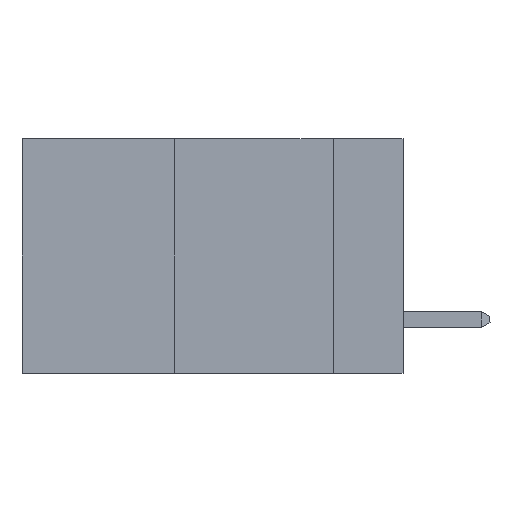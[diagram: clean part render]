
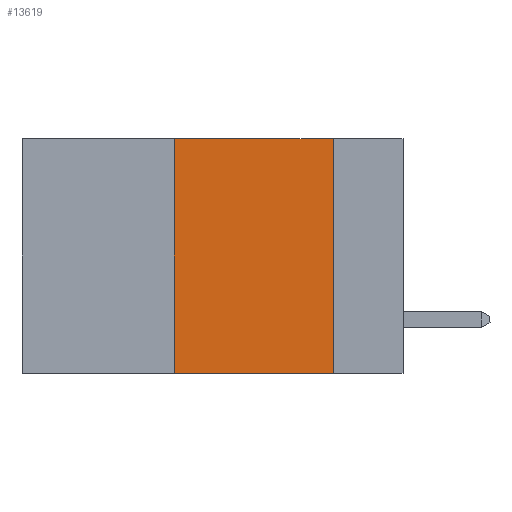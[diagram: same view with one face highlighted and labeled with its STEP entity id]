
A CAD part, left-side view. The second image highlights one B-rep face of the part: STEP entity #13619.
In plain terms, the highlighted planar face has unit normal (-1, 0, 0).
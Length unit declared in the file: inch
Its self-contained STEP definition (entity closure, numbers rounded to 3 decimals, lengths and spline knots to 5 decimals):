
#525 = DIRECTION ( 'NONE',  ( 1., 0., 0. ) ) ;
#1082 = ORIENTED_EDGE ( 'NONE', *, *, #5731, .F. ) ;
#1224 = ORIENTED_EDGE ( 'NONE', *, *, #4585, .F. ) ;
#1263 = ORIENTED_EDGE ( 'NONE', *, *, #1955, .F. ) ;
#1331 = ORIENTED_EDGE ( 'NONE', *, *, #15946, .T. ) ;
#1877 = LINE ( 'NONE', #10360, #13682 ) ;
#1931 = CARTESIAN_POINT ( 'NONE',  ( 0., 0.11, 0. ) ) ;
#1955 = EDGE_CURVE ( 'NONE', #7000, #3945, #12237, .T. ) ;
#1991 = DIRECTION ( 'NONE',  ( 0., -1., 0. ) ) ;
#2933 = AXIS2_PLACEMENT_3D ( 'NONE', #16819, #525, #10323 ) ;
#3236 = CARTESIAN_POINT ( 'NONE',  ( 0., 0.36, -0.37 ) ) ;
#3374 = FACE_OUTER_BOUND ( 'NONE', #6062, .T. ) ;
#3945 = VERTEX_POINT ( 'NONE', #11039 ) ;
#4585 = EDGE_CURVE ( 'NONE', #3945, #13025, #9209, .T. ) ;
#5635 = DIRECTION ( 'NONE',  ( 0., 0., 1. ) ) ;
#5731 = EDGE_CURVE ( 'NONE', #13025, #6872, #15547, .T. ) ;
#6062 = EDGE_LOOP ( 'NONE', ( #1082, #1224, #1263, #1331 ) ) ;
#6872 = VERTEX_POINT ( 'NONE', #16484 ) ;
#7000 = VERTEX_POINT ( 'NONE', #3236 ) ;
#8939 = PLANE ( 'NONE',  #2933 ) ;
#9209 = LINE ( 'NONE', #15872, #12745 ) ;
#9902 = CARTESIAN_POINT ( 'NONE',  ( 0., 0.36, 0. ) ) ;
#10323 = DIRECTION ( 'NONE',  ( 0., 0., -1. ) ) ;
#10360 = CARTESIAN_POINT ( 'NONE',  ( 0., 0.6, -0.37 ) ) ;
#11039 = CARTESIAN_POINT ( 'NONE',  ( 0., 0.36, 0. ) ) ;
#12016 = DIRECTION ( 'NONE',  ( 0., -1., 0. ) ) ;
#12237 = LINE ( 'NONE', #9902, #15274 ) ;
#12509 = VECTOR ( 'NONE', #12957, 39.37008 ) ;
#12745 = VECTOR ( 'NONE', #12016, 39.37008 ) ;
#12957 = DIRECTION ( 'NONE',  ( 0., 0., -1. ) ) ;
#13025 = VERTEX_POINT ( 'NONE', #16656 ) ;
#13619 = ADVANCED_FACE ( 'NONE', ( #3374 ), #8939, .F. ) ;
#13682 = VECTOR ( 'NONE', #1991, 39.37008 ) ;
#15274 = VECTOR ( 'NONE', #5635, 39.37008 ) ;
#15547 = LINE ( 'NONE', #1931, #12509 ) ;
#15872 = CARTESIAN_POINT ( 'NONE',  ( 0., 0.6, 0. ) ) ;
#15946 = EDGE_CURVE ( 'NONE', #7000, #6872, #1877, .T. ) ;
#16484 = CARTESIAN_POINT ( 'NONE',  ( 0., 0.11, -0.37 ) ) ;
#16656 = CARTESIAN_POINT ( 'NONE',  ( 0., 0.11, 0. ) ) ;
#16819 = CARTESIAN_POINT ( 'NONE',  ( 0., 0.6, 0. ) ) ;
